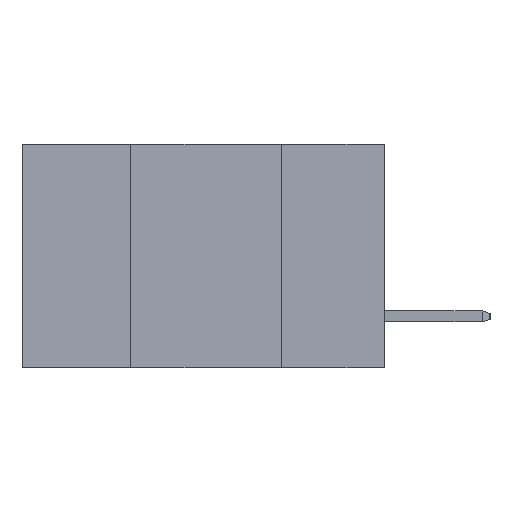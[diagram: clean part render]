
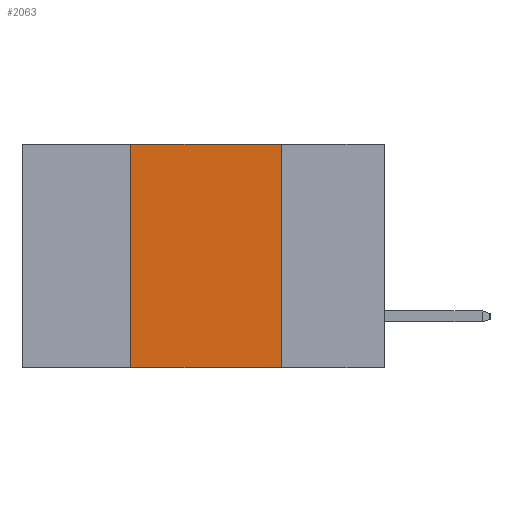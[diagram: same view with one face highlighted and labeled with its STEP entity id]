
A CAD part, left-side view. The second image highlights one B-rep face of the part: STEP entity #2063.
In plain terms, the highlighted planar face has unit normal (-1, 0, 0).
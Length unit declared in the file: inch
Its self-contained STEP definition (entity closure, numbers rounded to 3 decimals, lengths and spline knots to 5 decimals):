
#597 = ORIENTED_EDGE ( 'NONE', *, *, #5674, .T. ) ;
#745 = CARTESIAN_POINT ( 'NONE',  ( 0., 0.6, -0.37 ) ) ;
#1530 = DIRECTION ( 'NONE',  ( 0., 0., -1. ) ) ;
#1977 = VECTOR ( 'NONE', #12644, 39.37008 ) ;
#2063 = ADVANCED_FACE ( 'NONE', ( #16947 ), #16411, .F. ) ;
#2698 = CARTESIAN_POINT ( 'NONE',  ( 0., 0.17, 0. ) ) ;
#2907 = VECTOR ( 'NONE', #16717, 39.37008 ) ;
#3299 = DIRECTION ( 'NONE',  ( 0., 0., 1. ) ) ;
#3325 = EDGE_CURVE ( 'NONE', #7357, #13576, #12645, .T. ) ;
#4519 = VECTOR ( 'NONE', #10375, 39.37008 ) ;
#4588 = VERTEX_POINT ( 'NONE', #4944 ) ;
#4944 = CARTESIAN_POINT ( 'NONE',  ( 0., 0.42, -0.37 ) ) ;
#5194 = DIRECTION ( 'NONE',  ( 1., 0., 0. ) ) ;
#5674 = EDGE_CURVE ( 'NONE', #4588, #13576, #11262, .T. ) ;
#5733 = VECTOR ( 'NONE', #3299, 39.37008 ) ;
#7205 = ORIENTED_EDGE ( 'NONE', *, *, #16845, .F. ) ;
#7283 = ORIENTED_EDGE ( 'NONE', *, *, #3325, .F. ) ;
#7357 = VERTEX_POINT ( 'NONE', #2698 ) ;
#7503 = VERTEX_POINT ( 'NONE', #9882 ) ;
#9086 = CARTESIAN_POINT ( 'NONE',  ( 0., 0.6, 0. ) ) ;
#9827 = LINE ( 'NONE', #9086, #2907 ) ;
#9882 = CARTESIAN_POINT ( 'NONE',  ( 0., 0.42, 0. ) ) ;
#10167 = CARTESIAN_POINT ( 'NONE',  ( 0., 0.42, 0. ) ) ;
#10375 = DIRECTION ( 'NONE',  ( 0., -1., 0. ) ) ;
#11262 = LINE ( 'NONE', #745, #4519 ) ;
#11636 = AXIS2_PLACEMENT_3D ( 'NONE', #16956, #5194, #1530 ) ;
#12544 = EDGE_LOOP ( 'NONE', ( #7283, #16879, #7205, #597 ) ) ;
#12645 = LINE ( 'NONE', #13568, #1977 ) ;
#12644 = DIRECTION ( 'NONE',  ( 0., 0., -1. ) ) ;
#13247 = EDGE_CURVE ( 'NONE', #7503, #7357, #9827, .T. ) ;
#13568 = CARTESIAN_POINT ( 'NONE',  ( 0., 0.17, 0. ) ) ;
#13576 = VERTEX_POINT ( 'NONE', #13704 ) ;
#13704 = CARTESIAN_POINT ( 'NONE',  ( 0., 0.17, -0.37 ) ) ;
#16411 = PLANE ( 'NONE',  #11636 ) ;
#16570 = LINE ( 'NONE', #10167, #5733 ) ;
#16717 = DIRECTION ( 'NONE',  ( 0., -1., 0. ) ) ;
#16845 = EDGE_CURVE ( 'NONE', #4588, #7503, #16570, .T. ) ;
#16879 = ORIENTED_EDGE ( 'NONE', *, *, #13247, .F. ) ;
#16947 = FACE_OUTER_BOUND ( 'NONE', #12544, .T. ) ;
#16956 = CARTESIAN_POINT ( 'NONE',  ( 0., 0.6, 0. ) ) ;
